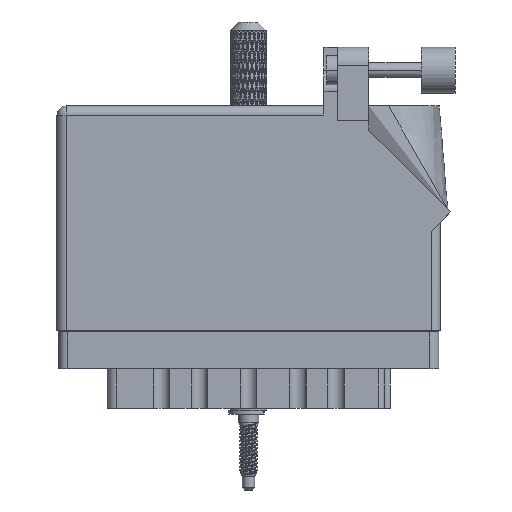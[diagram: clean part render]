
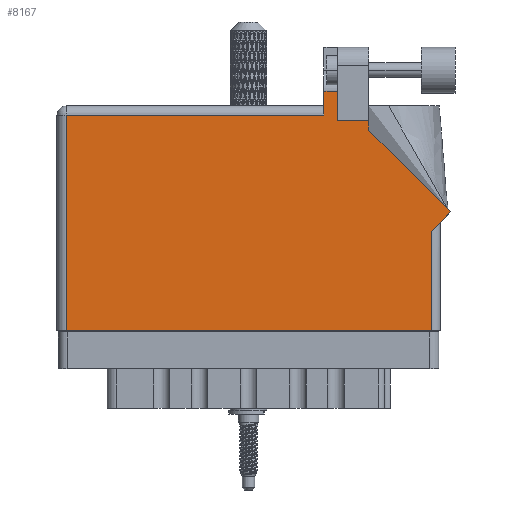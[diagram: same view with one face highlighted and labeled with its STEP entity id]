
A CAD part, front view. The second image highlights one B-rep face of the part: STEP entity #8167.
In plain terms, the highlighted face is planar.
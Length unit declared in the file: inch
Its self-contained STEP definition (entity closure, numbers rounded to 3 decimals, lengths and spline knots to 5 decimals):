
#3086 = DIRECTION ( 'NONE',  ( -1., 0., 0. ) ) ;
#7986 = CARTESIAN_POINT ( 'NONE',  ( 2.55, 0.737, 0. ) ) ;
#8167 = ADVANCED_FACE ( 'NONE', ( #47863 ), #58733, .F. ) ;
#8835 = LINE ( 'NONE', #100248, #65678 ) ;
#9370 = ORIENTED_EDGE ( 'NONE', *, *, #33855, .T. ) ;
#9453 = ORIENTED_EDGE ( 'NONE', *, *, #59424, .T. ) ;
#9950 = CARTESIAN_POINT ( 'NONE',  ( 1.819, 1.53, 0. ) ) ;
#11552 = DIRECTION ( 'NONE',  ( 0., 0., -1. ) ) ;
#11904 = VECTOR ( 'NONE', #92005, 39.37008 ) ;
#11916 = CARTESIAN_POINT ( 'NONE',  ( 2.24377, 1.6315, 0. ) ) ;
#12194 = CARTESIAN_POINT ( 'NONE',  ( 0.062, 1.468, 0. ) ) ;
#12285 = DIRECTION ( 'NONE',  ( 0., 1., 0. ) ) ;
#12903 = CARTESIAN_POINT ( 'NONE',  ( 2.612, 0.737, 0. ) ) ;
#15087 = ORIENTED_EDGE ( 'NONE', *, *, #100408, .T. ) ;
#15262 = VERTEX_POINT ( 'NONE', #32492 ) ;
#15406 = EDGE_LOOP ( 'NONE', ( #73086, #9453, #15087, #95369, #9370, #27271, #62244, #113734, #89864, #108299, #75717 ) ) ;
#16299 = CARTESIAN_POINT ( 'NONE',  ( 2.126, 1.36442, 0. ) ) ;
#19983 = CARTESIAN_POINT ( 'NONE',  ( 2.126, 1.43, 0. ) ) ;
#20837 = LINE ( 'NONE', #9950, #42650 ) ;
#21278 = VECTOR ( 'NONE', #54050, 39.37008 ) ;
#22796 = LINE ( 'NONE', #11916, #43027 ) ;
#23539 = VERTEX_POINT ( 'NONE', #12194 ) ;
#23958 = VECTOR ( 'NONE', #75061, 39.37008 ) ;
#24858 = DIRECTION ( 'NONE',  ( -1., 0., 0. ) ) ;
#26733 = EDGE_CURVE ( 'NONE', #93138, #23539, #49880, .T. ) ;
#27271 = ORIENTED_EDGE ( 'NONE', *, *, #49594, .T. ) ;
#32492 = CARTESIAN_POINT ( 'NONE',  ( 2.55, 0.675, 0. ) ) ;
#32718 = CARTESIAN_POINT ( 'NONE',  ( 1.913, 1.43, 0. ) ) ;
#32827 = DIRECTION ( 'NONE',  ( 0.707, 0.707, 0. ) ) ;
#33023 = DIRECTION ( 'NONE',  ( 0., 1., 0. ) ) ;
#33855 = EDGE_CURVE ( 'NONE', #23539, #113176, #81315, .T. ) ;
#34495 = VERTEX_POINT ( 'NONE', #62685 ) ;
#40800 = CARTESIAN_POINT ( 'NONE',  ( 0., 1.468, 0. ) ) ;
#41031 = VERTEX_POINT ( 'NONE', #16299 ) ;
#41367 = CARTESIAN_POINT ( 'NONE',  ( 1.913, 1.6315, 0. ) ) ;
#42650 = VECTOR ( 'NONE', #92283, 39.37008 ) ;
#43027 = VECTOR ( 'NONE', #85770, 39.37008 ) ;
#43511 = CARTESIAN_POINT ( 'NONE',  ( 1.819, 1.6315, 0. ) ) ;
#47863 = FACE_OUTER_BOUND ( 'NONE', #15406, .T. ) ;
#48604 = LINE ( 'NONE', #85533, #97358 ) ;
#49594 = EDGE_CURVE ( 'NONE', #113176, #34495, #8835, .T. ) ;
#49880 = LINE ( 'NONE', #40800, #73002 ) ;
#50034 = EDGE_CURVE ( 'NONE', #15262, #66447, #95835, .T. ) ;
#50341 = LINE ( 'NONE', #115765, #59179 ) ;
#52962 = VERTEX_POINT ( 'NONE', #43511 ) ;
#53268 = CARTESIAN_POINT ( 'NONE',  ( 2.126, 1.36442, 0. ) ) ;
#54050 = DIRECTION ( 'NONE',  ( 0., -1., 0. ) ) ;
#55083 = LINE ( 'NONE', #74461, #23958 ) ;
#58733 = PLANE ( 'NONE',  #104967 ) ;
#59179 = VECTOR ( 'NONE', #24858, 39.37008 ) ;
#59424 = EDGE_CURVE ( 'NONE', #90181, #52962, #22796, .T. ) ;
#61091 = EDGE_CURVE ( 'NONE', #66447, #41031, #55083, .T. ) ;
#62244 = ORIENTED_EDGE ( 'NONE', *, *, #73455, .T. ) ;
#62685 = CARTESIAN_POINT ( 'NONE',  ( 2.55, 0., 0. ) ) ;
#65678 = VECTOR ( 'NONE', #110576, 39.37008 ) ;
#66447 = VERTEX_POINT ( 'NONE', #81964 ) ;
#68083 = CARTESIAN_POINT ( 'NONE',  ( 1.819, 1.468, 0. ) ) ;
#73002 = VECTOR ( 'NONE', #115892, 39.37008 ) ;
#73086 = ORIENTED_EDGE ( 'NONE', *, *, #106458, .T. ) ;
#73455 = EDGE_CURVE ( 'NONE', #34495, #15262, #90922, .T. ) ;
#74461 = CARTESIAN_POINT ( 'NONE',  ( 2.68271, 0.80771, 0. ) ) ;
#75061 = DIRECTION ( 'NONE',  ( -0.707, 0.707, 0. ) ) ;
#75717 = ORIENTED_EDGE ( 'NONE', *, *, #83145, .T. ) ;
#79319 = VERTEX_POINT ( 'NONE', #32718 ) ;
#81315 = LINE ( 'NONE', #99484, #21278 ) ;
#81964 = CARTESIAN_POINT ( 'NONE',  ( 2.68271, 0.80771, 0. ) ) ;
#83145 = EDGE_CURVE ( 'NONE', #83344, #79319, #50341, .T. ) ;
#83344 = VERTEX_POINT ( 'NONE', #19983 ) ;
#85533 = CARTESIAN_POINT ( 'NONE',  ( 1.913, 1.43, 0. ) ) ;
#85770 = DIRECTION ( 'NONE',  ( -1., 0., 0. ) ) ;
#89864 = ORIENTED_EDGE ( 'NONE', *, *, #61091, .T. ) ;
#90181 = VERTEX_POINT ( 'NONE', #41367 ) ;
#90922 = LINE ( 'NONE', #7986, #95087 ) ;
#92005 = DIRECTION ( 'NONE',  ( 0., 1., 0. ) ) ;
#92283 = DIRECTION ( 'NONE',  ( 0., -1., 0. ) ) ;
#93138 = VERTEX_POINT ( 'NONE', #68083 ) ;
#95087 = VECTOR ( 'NONE', #33023, 39.37008 ) ;
#95369 = ORIENTED_EDGE ( 'NONE', *, *, #26733, .T. ) ;
#95835 = LINE ( 'NONE', #12903, #96760 ) ;
#96760 = VECTOR ( 'NONE', #32827, 39.37008 ) ;
#97358 = VECTOR ( 'NONE', #12285, 39.37008 ) ;
#97393 = CARTESIAN_POINT ( 'NONE',  ( 0.062, 0., 0. ) ) ;
#99279 = LINE ( 'NONE', #53268, #11904 ) ;
#99484 = CARTESIAN_POINT ( 'NONE',  ( 0.062, 0., 0. ) ) ;
#100248 = CARTESIAN_POINT ( 'NONE',  ( 0., 0., 0. ) ) ;
#100408 = EDGE_CURVE ( 'NONE', #52962, #93138, #20837, .T. ) ;
#103318 = EDGE_CURVE ( 'NONE', #41031, #83344, #99279, .T. ) ;
#104169 = CARTESIAN_POINT ( 'NONE',  ( 0., 1.53, 0. ) ) ;
#104967 = AXIS2_PLACEMENT_3D ( 'NONE', #104169, #11552, #3086 ) ;
#106458 = EDGE_CURVE ( 'NONE', #79319, #90181, #48604, .T. ) ;
#108299 = ORIENTED_EDGE ( 'NONE', *, *, #103318, .T. ) ;
#110576 = DIRECTION ( 'NONE',  ( 1., 0., 0. ) ) ;
#113176 = VERTEX_POINT ( 'NONE', #97393 ) ;
#113734 = ORIENTED_EDGE ( 'NONE', *, *, #50034, .T. ) ;
#115765 = CARTESIAN_POINT ( 'NONE',  ( 2.126, 1.43, 0. ) ) ;
#115892 = DIRECTION ( 'NONE',  ( -1., 0., 0. ) ) ;
